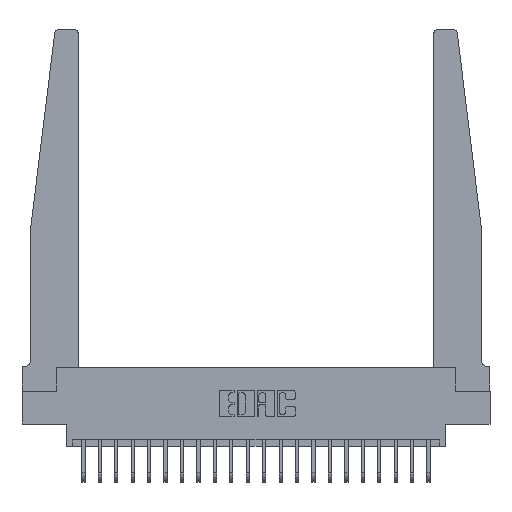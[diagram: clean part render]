
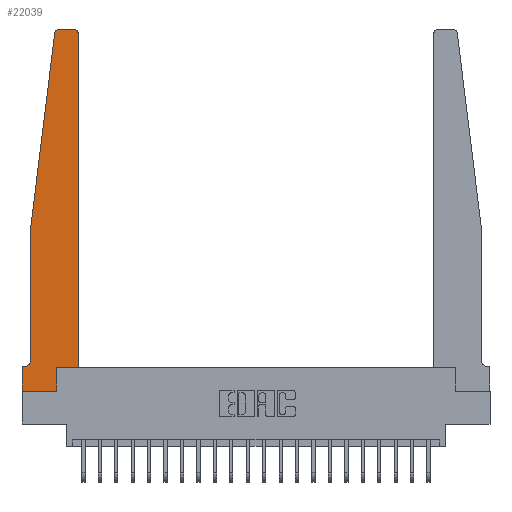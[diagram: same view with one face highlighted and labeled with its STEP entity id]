
A CAD part, top view. The second image highlights one B-rep face of the part: STEP entity #22039.
In plain terms, the highlighted planar face has unit normal (0, 0, 1).
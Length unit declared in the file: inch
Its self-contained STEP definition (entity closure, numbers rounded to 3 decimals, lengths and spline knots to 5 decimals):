
#338 = EDGE_CURVE ( 'NONE', #14819, #2730, #14077, .T. ) ;
#526 = DIRECTION ( 'NONE',  ( 0., 0., -1. ) ) ;
#731 = LINE ( 'NONE', #6752, #5029 ) ;
#774 = ORIENTED_EDGE ( 'NONE', *, *, #19113, .T. ) ;
#806 = CARTESIAN_POINT ( 'NONE',  ( 0., 0.1875, 0.37 ) ) ;
#1060 = VECTOR ( 'NONE', #7238, 39.37008 ) ;
#1290 = VERTEX_POINT ( 'NONE', #19604 ) ;
#1523 = AXIS2_PLACEMENT_3D ( 'NONE', #806, #15268, #8169 ) ;
#2380 = ORIENTED_EDGE ( 'NONE', *, *, #12102, .T. ) ;
#2478 = CARTESIAN_POINT ( 'NONE',  ( 0.065, 0.1875, 0.37 ) ) ;
#2502 = CARTESIAN_POINT ( 'NONE',  ( 0.24675, 2.72367, 0.37 ) ) ;
#2730 = VERTEX_POINT ( 'NONE', #14214 ) ;
#2940 = LINE ( 'NONE', #18600, #16419 ) ;
#3114 = VERTEX_POINT ( 'NONE', #22187 ) ;
#3265 = ORIENTED_EDGE ( 'NONE', *, *, #18420, .T. ) ;
#3585 = EDGE_CURVE ( 'NONE', #2730, #14011, #13789, .T. ) ;
#4029 = ORIENTED_EDGE ( 'NONE', *, *, #9757, .T. ) ;
#4233 = CARTESIAN_POINT ( 'NONE',  ( 0.015, 0.2375, 0.37 ) ) ;
#4433 = EDGE_CURVE ( 'NONE', #18449, #16320, #21212, .T. ) ;
#4548 = AXIS2_PLACEMENT_3D ( 'NONE', #4233, #526, #7667 ) ;
#4603 = VERTEX_POINT ( 'NONE', #17305 ) ;
#4658 = DIRECTION ( 'NONE',  ( 1., 0., 0. ) ) ;
#5029 = VECTOR ( 'NONE', #8578, 39.37008 ) ;
#5248 = CARTESIAN_POINT ( 'NONE',  ( 0., 0., 0.37 ) ) ;
#6295 = EDGE_CURVE ( 'NONE', #1290, #14819, #18870, .T. ) ;
#6377 = ORIENTED_EDGE ( 'NONE', *, *, #9702, .T. ) ;
#6752 = CARTESIAN_POINT ( 'NONE',  ( 0., 0., 0.37 ) ) ;
#7238 = DIRECTION ( 'NONE',  ( 0., 1., 0. ) ) ;
#7575 = CARTESIAN_POINT ( 'NONE',  ( 0.395, 2.72, 0.37 ) ) ;
#7667 = DIRECTION ( 'NONE',  ( -1., 0., 0. ) ) ;
#7683 = CARTESIAN_POINT ( 'NONE',  ( 0.065, 1.25, 0.37 ) ) ;
#7737 = ORIENTED_EDGE ( 'NONE', *, *, #3585, .T. ) ;
#7894 = VERTEX_POINT ( 'NONE', #20918 ) ;
#8169 = DIRECTION ( 'NONE',  ( 1., 0., 0. ) ) ;
#8504 = ORIENTED_EDGE ( 'NONE', *, *, #19465, .T. ) ;
#8578 = DIRECTION ( 'NONE',  ( 0., -1., 0. ) ) ;
#8842 = EDGE_CURVE ( 'NONE', #16310, #20079, #731, .T. ) ;
#9126 = CARTESIAN_POINT ( 'NONE',  ( 0.27653, 2.72, 0.37 ) ) ;
#9419 = DIRECTION ( 'NONE',  ( 1., 0., 0. ) ) ;
#9495 = CARTESIAN_POINT ( 'NONE',  ( 0.425, 0.18, 0.37 ) ) ;
#9616 = CARTESIAN_POINT ( 'NONE',  ( 0.065, 1.25, 0.37 ) ) ;
#9702 = EDGE_CURVE ( 'NONE', #14011, #4603, #10355, .T. ) ;
#9757 = EDGE_CURVE ( 'NONE', #4603, #14965, #2940, .T. ) ;
#10020 = PLANE ( 'NONE',  #1523 ) ;
#10299 = VECTOR ( 'NONE', #23510, 39.37008 ) ;
#10355 = CIRCLE ( 'NONE', #19556, 0.03 ) ;
#11372 = CARTESIAN_POINT ( 'NONE',  ( 0., 0.1875, 0.37 ) ) ;
#12102 = EDGE_CURVE ( 'NONE', #14965, #18449, #23755, .T. ) ;
#12647 = DIRECTION ( 'NONE',  ( 1., 0., 0. ) ) ;
#13789 = LINE ( 'NONE', #9495, #14061 ) ;
#13901 = AXIS2_PLACEMENT_3D ( 'NONE', #9126, #19905, #12647 ) ;
#14011 = VERTEX_POINT ( 'NONE', #17430 ) ;
#14061 = VECTOR ( 'NONE', #18743, 39.37008 ) ;
#14077 = LINE ( 'NONE', #21114, #20132 ) ;
#14214 = CARTESIAN_POINT ( 'NONE',  ( 0.425, 0.18, 0.37 ) ) ;
#14476 = CARTESIAN_POINT ( 'NONE',  ( 0.2605, 0.18, 0.37 ) ) ;
#14819 = VERTEX_POINT ( 'NONE', #20599 ) ;
#14965 = VERTEX_POINT ( 'NONE', #21638 ) ;
#15268 = DIRECTION ( 'NONE',  ( 0., 0., 1. ) ) ;
#15315 = EDGE_LOOP ( 'NONE', ( #4029, #2380, #21365, #3265, #21002, #774, #21104, #8504, #18128, #17040, #7737, #6377 ) ) ;
#15797 = LINE ( 'NONE', #9616, #19241 ) ;
#16310 = VERTEX_POINT ( 'NONE', #11372 ) ;
#16320 = VERTEX_POINT ( 'NONE', #7683 ) ;
#16419 = VECTOR ( 'NONE', #17164, 39.37008 ) ;
#16633 = VECTOR ( 'NONE', #18995, 39.37008 ) ;
#17040 = ORIENTED_EDGE ( 'NONE', *, *, #338, .T. ) ;
#17164 = DIRECTION ( 'NONE',  ( -1., 0., 0. ) ) ;
#17219 = CARTESIAN_POINT ( 'NONE',  ( 0.065, 1.25, 0.37 ) ) ;
#17246 = VECTOR ( 'NONE', #22770, 39.37008 ) ;
#17305 = CARTESIAN_POINT ( 'NONE',  ( 0.395, 2.75, 0.37 ) ) ;
#17430 = CARTESIAN_POINT ( 'NONE',  ( 0.425, 2.72, 0.37 ) ) ;
#18128 = ORIENTED_EDGE ( 'NONE', *, *, #6295, .T. ) ;
#18420 = EDGE_CURVE ( 'NONE', #16320, #7894, #15797, .T. ) ;
#18449 = VERTEX_POINT ( 'NONE', #2502 ) ;
#18600 = CARTESIAN_POINT ( 'NONE',  ( 0.25, 2.75, 0.37 ) ) ;
#18743 = DIRECTION ( 'NONE',  ( 0., 1., 0. ) ) ;
#18870 = LINE ( 'NONE', #14476, #1060 ) ;
#18995 = DIRECTION ( 'NONE',  ( -1., 0., 0. ) ) ;
#19030 = EDGE_CURVE ( 'NONE', #7894, #3114, #22921, .T. ) ;
#19113 = EDGE_CURVE ( 'NONE', #3114, #16310, #20349, .T. ) ;
#19241 = VECTOR ( 'NONE', #20868, 39.37008 ) ;
#19465 = EDGE_CURVE ( 'NONE', #20079, #1290, #20050, .T. ) ;
#19556 = AXIS2_PLACEMENT_3D ( 'NONE', #7575, #22252, #9419 ) ;
#19604 = CARTESIAN_POINT ( 'NONE',  ( 0.2605, 0., 0.37 ) ) ;
#19905 = DIRECTION ( 'NONE',  ( 0., 0., 1. ) ) ;
#19973 = FACE_OUTER_BOUND ( 'NONE', #15315, .T. ) ;
#20050 = LINE ( 'NONE', #5248, #10299 ) ;
#20079 = VERTEX_POINT ( 'NONE', #23313 ) ;
#20132 = VECTOR ( 'NONE', #4658, 39.37008 ) ;
#20349 = LINE ( 'NONE', #2478, #16633 ) ;
#20599 = CARTESIAN_POINT ( 'NONE',  ( 0.2605, 0.18, 0.37 ) ) ;
#20868 = DIRECTION ( 'NONE',  ( 0., -1., 0. ) ) ;
#20918 = CARTESIAN_POINT ( 'NONE',  ( 0.065, 0.2375, 0.37 ) ) ;
#21002 = ORIENTED_EDGE ( 'NONE', *, *, #19030, .T. ) ;
#21104 = ORIENTED_EDGE ( 'NONE', *, *, #8842, .T. ) ;
#21114 = CARTESIAN_POINT ( 'NONE',  ( 0.425, 0.18, 0.37 ) ) ;
#21212 = LINE ( 'NONE', #17219, #17246 ) ;
#21365 = ORIENTED_EDGE ( 'NONE', *, *, #4433, .T. ) ;
#21638 = CARTESIAN_POINT ( 'NONE',  ( 0.27653, 2.75, 0.37 ) ) ;
#22039 = ADVANCED_FACE ( 'NONE', ( #19973 ), #10020, .T. ) ;
#22187 = CARTESIAN_POINT ( 'NONE',  ( 0.015, 0.1875, 0.37 ) ) ;
#22252 = DIRECTION ( 'NONE',  ( 0., 0., 1. ) ) ;
#22770 = DIRECTION ( 'NONE',  ( -0.122, -0.992, 0. ) ) ;
#22921 = CIRCLE ( 'NONE', #4548, 0.05 ) ;
#23313 = CARTESIAN_POINT ( 'NONE',  ( 0., 0., 0.37 ) ) ;
#23510 = DIRECTION ( 'NONE',  ( 1., 0., 0. ) ) ;
#23755 = CIRCLE ( 'NONE', #13901, 0.03 ) ;
